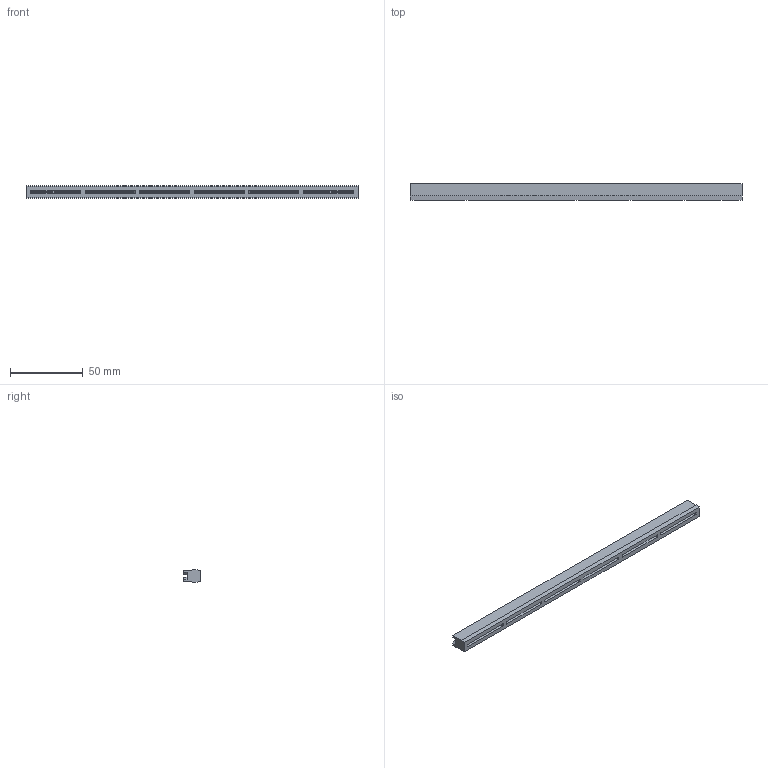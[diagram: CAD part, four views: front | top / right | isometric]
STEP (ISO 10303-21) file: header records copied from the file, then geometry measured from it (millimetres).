
FILE_DESCRIPTION (( 'STEP AP214' ), '1' );
FILE_NAME ('616-220-312.STEP', '2020-08-20T18:15:52', ( '' ), ( '' ), 'SwSTEP 2.0', 'SolidWorks 2020', '' );
FILE_SCHEMA (( 'AUTOMOTIVE_DESIGN' ));
Length unit declared in the file: inch
Products named in the file (1): 616-220-312
Bounding box: 228.6 x 11.68 x 8.38 mm (x, y, z)
Volume: 18298.1 mm3; surface area: 12784.1 mm2
Topology: 1 solids, 1 shells, 291 faces, 741 edges, 454 vertices
Faces by surface type: plane 144, bspline 75, cylinder 48, sphere 24
Entity records: 12849 total; most frequent: CARTESIAN_POINT 6482, ORIENTED_EDGE 1434, DIRECTION 1049, EDGE_CURVE 717, LINE 471, VECTOR 471, VERTEX_POINT 454, EDGE_LOOP 317
